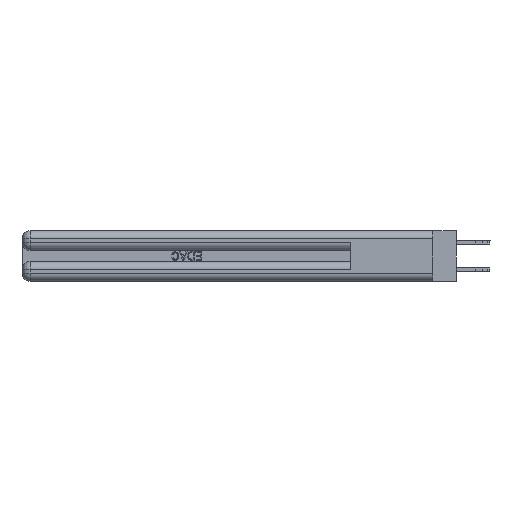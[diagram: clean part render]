
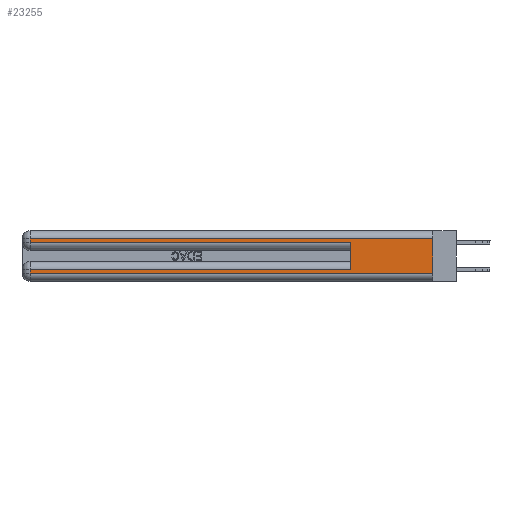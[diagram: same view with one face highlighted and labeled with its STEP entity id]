
A CAD part, left-side view. The second image highlights one B-rep face of the part: STEP entity #23255.
In plain terms, the highlighted planar face has unit normal (-1, 0, 0).
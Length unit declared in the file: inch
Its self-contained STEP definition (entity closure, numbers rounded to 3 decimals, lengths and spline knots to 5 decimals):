
#730 = CARTESIAN_POINT ( 'NONE',  ( 0., 0., 0.31 ) ) ;
#1015 = CARTESIAN_POINT ( 'NONE',  ( 0., 0., 0.37 ) ) ;
#1341 = LINE ( 'NONE', #31019, #6449 ) ;
#1906 = EDGE_CURVE ( 'NONE', #20226, #36858, #20567, .T. ) ;
#2246 = CARTESIAN_POINT ( 'NONE',  ( 0., 2.94, 0.37 ) ) ;
#3157 = VECTOR ( 'NONE', #41335, 39.37008 ) ;
#3491 = FACE_OUTER_BOUND ( 'NONE', #26578, .T. ) ;
#4440 = VERTEX_POINT ( 'NONE', #28124 ) ;
#4915 = VERTEX_POINT ( 'NONE', #22784 ) ;
#5278 = ORIENTED_EDGE ( 'NONE', *, *, #1906, .F. ) ;
#5516 = LINE ( 'NONE', #31521, #39066 ) ;
#5709 = LINE ( 'NONE', #2246, #3157 ) ;
#6449 = VECTOR ( 'NONE', #37694, 39.37008 ) ;
#7599 = CARTESIAN_POINT ( 'NONE',  ( 0., 2.94, 0.31 ) ) ;
#7697 = LINE ( 'NONE', #36902, #23439 ) ;
#8169 = LINE ( 'NONE', #12638, #41214 ) ;
#8671 = ORIENTED_EDGE ( 'NONE', *, *, #32420, .T. ) ;
#8799 = DIRECTION ( 'NONE',  ( 0., 1., 0. ) ) ;
#9916 = ORIENTED_EDGE ( 'NONE', *, *, #17967, .T. ) ;
#10534 = ORIENTED_EDGE ( 'NONE', *, *, #28820, .T. ) ;
#11187 = VECTOR ( 'NONE', #22093, 39.37008 ) ;
#11655 = DIRECTION ( 'NONE',  ( 0., 0., -1. ) ) ;
#11775 = CARTESIAN_POINT ( 'NONE',  ( 0., 2.94, 0.085 ) ) ;
#12079 = LINE ( 'NONE', #13015, #13640 ) ;
#12638 = CARTESIAN_POINT ( 'NONE',  ( 0., 0., 0.31 ) ) ;
#12903 = VECTOR ( 'NONE', #11655, 39.37008 ) ;
#13015 = CARTESIAN_POINT ( 'NONE',  ( 0., 0., 0.285 ) ) ;
#13640 = VECTOR ( 'NONE', #19581, 39.37008 ) ;
#15046 = ORIENTED_EDGE ( 'NONE', *, *, #24244, .T. ) ;
#17113 = DIRECTION ( 'NONE',  ( 0., 0., -1. ) ) ;
#17588 = AXIS2_PLACEMENT_3D ( 'NONE', #36312, #26767, #17113 ) ;
#17599 = ORIENTED_EDGE ( 'NONE', *, *, #31508, .T. ) ;
#17967 = EDGE_CURVE ( 'NONE', #23156, #36858, #5516, .T. ) ;
#18981 = EDGE_CURVE ( 'NONE', #4915, #4440, #1341, .T. ) ;
#19581 = DIRECTION ( 'NONE',  ( 0., -1., 0. ) ) ;
#19704 = DIRECTION ( 'NONE',  ( 0., -1., 0. ) ) ;
#20226 = VERTEX_POINT ( 'NONE', #730 ) ;
#20247 = PLANE ( 'NONE',  #17588 ) ;
#20567 = LINE ( 'NONE', #1015, #12903 ) ;
#22093 = DIRECTION ( 'NONE',  ( 0., 1., 0. ) ) ;
#22701 = ORIENTED_EDGE ( 'NONE', *, *, #31957, .T. ) ;
#22784 = CARTESIAN_POINT ( 'NONE',  ( 0., 0.6, 0.085 ) ) ;
#23156 = VERTEX_POINT ( 'NONE', #32377 ) ;
#23255 = ADVANCED_FACE ( 'NONE', ( #3491 ), #20247, .F. ) ;
#23439 = VECTOR ( 'NONE', #40161, 39.37008 ) ;
#24151 = ORIENTED_EDGE ( 'NONE', *, *, #18981, .F. ) ;
#24244 = EDGE_CURVE ( 'NONE', #28504, #4440, #12079, .T. ) ;
#24993 = VERTEX_POINT ( 'NONE', #7599 ) ;
#25765 = VERTEX_POINT ( 'NONE', #11775 ) ;
#26578 = EDGE_LOOP ( 'NONE', ( #5278, #8671, #17599, #15046, #24151, #10534, #22701, #9916 ) ) ;
#26767 = DIRECTION ( 'NONE',  ( 1., 0., 0. ) ) ;
#27109 = CARTESIAN_POINT ( 'NONE',  ( 0., 2.94, 0.285 ) ) ;
#28124 = CARTESIAN_POINT ( 'NONE',  ( 0., 0.6, 0.285 ) ) ;
#28504 = VERTEX_POINT ( 'NONE', #27109 ) ;
#28820 = EDGE_CURVE ( 'NONE', #4915, #25765, #32035, .T. ) ;
#31019 = CARTESIAN_POINT ( 'NONE',  ( 0., 0.6, 0.145 ) ) ;
#31508 = EDGE_CURVE ( 'NONE', #24993, #28504, #5709, .T. ) ;
#31521 = CARTESIAN_POINT ( 'NONE',  ( 0., 0., 0.06 ) ) ;
#31957 = EDGE_CURVE ( 'NONE', #25765, #23156, #7697, .T. ) ;
#32035 = LINE ( 'NONE', #35318, #11187 ) ;
#32377 = CARTESIAN_POINT ( 'NONE',  ( 0., 2.94, 0.06 ) ) ;
#32420 = EDGE_CURVE ( 'NONE', #20226, #24993, #8169, .T. ) ;
#35318 = CARTESIAN_POINT ( 'NONE',  ( 0., 0., 0.085 ) ) ;
#36312 = CARTESIAN_POINT ( 'NONE',  ( 0., 0., 0.37 ) ) ;
#36858 = VERTEX_POINT ( 'NONE', #39827 ) ;
#36902 = CARTESIAN_POINT ( 'NONE',  ( 0., 2.94, 0.37 ) ) ;
#37694 = DIRECTION ( 'NONE',  ( 0., 0., 1. ) ) ;
#39066 = VECTOR ( 'NONE', #19704, 39.37008 ) ;
#39827 = CARTESIAN_POINT ( 'NONE',  ( 0., 0., 0.06 ) ) ;
#40161 = DIRECTION ( 'NONE',  ( 0., 0., -1. ) ) ;
#41214 = VECTOR ( 'NONE', #8799, 39.37008 ) ;
#41335 = DIRECTION ( 'NONE',  ( 0., 0., -1. ) ) ;
